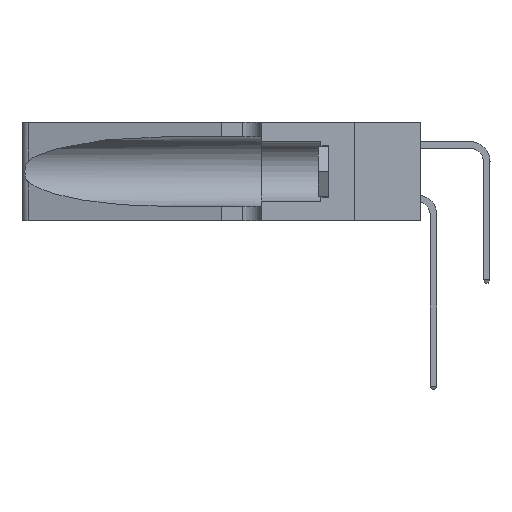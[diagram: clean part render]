
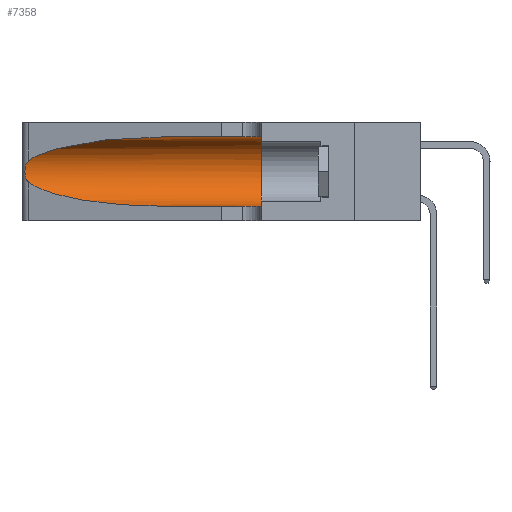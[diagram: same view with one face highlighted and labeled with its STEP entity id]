
A CAD part, left-side view. The second image highlights one B-rep face of the part: STEP entity #7358.
In plain terms, the highlighted cylindrical face has radius 3.308 mm (diameter 6.617 mm), a partial arc.
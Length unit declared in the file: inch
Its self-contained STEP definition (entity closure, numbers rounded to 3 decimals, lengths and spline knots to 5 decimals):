
#191 = ORIENTED_EDGE ( 'NONE', *, *, #30426, .T. ) ;
#884 = ORIENTED_EDGE ( 'NONE', *, *, #35435, .T. ) ;
#1092 = CARTESIAN_POINT ( 'NONE',  ( 0.25856, 1.23593, 0.16098 ) ) ;
#1130 = LINE ( 'NONE', #33942, #11367 ) ;
#1368 = LINE ( 'NONE', #7147, #33151 ) ;
#1555 = DIRECTION ( 'NONE',  ( 0., -1., 0. ) ) ;
#2728 = CYLINDRICAL_SURFACE ( 'NONE', #17965, 0.13025 ) ;
#3986 = CARTESIAN_POINT ( 'NONE',  ( 0.18966, 0.96281, 0.05475 ) ) ;
#5054 = EDGE_LOOP ( 'NONE', ( #191, #884, #16567, #29701, #20101, #30596 ) ) ;
#5937 = CIRCLE ( 'NONE', #17934, 0.13025 ) ;
#7131 = VERTEX_POINT ( 'NONE', #27624 ) ;
#7147 = CARTESIAN_POINT ( 'NONE',  ( 0.1305, 1.61858, 0.05475 ) ) ;
#7358 = ADVANCED_FACE ( 'NONE', ( #21085 ), #2728, .F. ) ;
#7449 = CARTESIAN_POINT ( 'NONE',  ( 0.2373, 1.15595, 0.08982 ) ) ;
#9213 =( BOUNDED_CURVE ( )  B_SPLINE_CURVE ( 3, ( #38783, #7449, #3986, #41925 ),
 .UNSPECIFIED., .F., .F. ) 
 B_SPLINE_CURVE_WITH_KNOTS ( ( 4, 4 ),
 ( 3.44316, 4.71239 ),
 .UNSPECIFIED. ) 
 CURVE ( )  GEOMETRIC_REPRESENTATION_ITEM ( )  RATIONAL_B_SPLINE_CURVE ( ( 1., 0.87, 0.87, 1. ) ) 
 REPRESENTATION_ITEM ( '' )  );
#9512 = DIRECTION ( 'NONE',  ( 0., 1., 0. ) ) ;
#11367 = VECTOR ( 'NONE', #26841, 39.37008 ) ;
#11779 = CARTESIAN_POINT ( 'NONE',  ( 0.25789, 1.23486, 0.15765 ) ) ;
#11877 = B_SPLINE_CURVE_WITH_KNOTS ( 'NONE', 3,
 ( #24388, #38260, #38575, #17968, #38730, #18113, #17671, #42181, #21100, #1092, #11779, #25757, #35576, #42627 ),
 .UNSPECIFIED., .F., .F.,
 ( 4, 2, 2, 2, 2, 2, 4 ),
 ( 0., 0.00027, 0.00053, 0.00107, 0.0016, 0.00187, 0.00214 ),
 .UNSPECIFIED. ) ;
#12684 = EDGE_CURVE ( 'NONE', #18525, #7131, #9213, .T. ) ;
#16567 = ORIENTED_EDGE ( 'NONE', *, *, #12684, .T. ) ;
#16637 = CARTESIAN_POINT ( 'NONE',  ( 0.18966, 0.96281, 0.31525 ) ) ;
#17388 = CARTESIAN_POINT ( 'NONE',  ( 0.25487, 1.22718, 0.22369 ) ) ;
#17671 = CARTESIAN_POINT ( 'NONE',  ( 0.26075, 1.23896, 0.19203 ) ) ;
#17934 = AXIS2_PLACEMENT_3D ( 'NONE', #23655, #9512, #23350 ) ;
#17965 = AXIS2_PLACEMENT_3D ( 'NONE', #39500, #1555, #42969 ) ;
#17968 = CARTESIAN_POINT ( 'NONE',  ( 0.25787, 1.23484, 0.2124 ) ) ;
#18113 = CARTESIAN_POINT ( 'NONE',  ( 0.26018, 1.23835, 0.19895 ) ) ;
#18525 = VERTEX_POINT ( 'NONE', #30726 ) ;
#20101 = ORIENTED_EDGE ( 'NONE', *, *, #28660, .F. ) ;
#21085 = FACE_OUTER_BOUND ( 'NONE', #5054, .T. ) ;
#21093 = EDGE_CURVE ( 'NONE', #7131, #40028, #1368, .T. ) ;
#21100 = CARTESIAN_POINT ( 'NONE',  ( 0.26017, 1.23833, 0.17102 ) ) ;
#23350 = DIRECTION ( 'NONE',  ( 0., 0., 1. ) ) ;
#23655 = CARTESIAN_POINT ( 'NONE',  ( 0.1305, 0.35, 0.185 ) ) ;
#23935 = VERTEX_POINT ( 'NONE', #41813 ) ;
#24388 = CARTESIAN_POINT ( 'NONE',  ( 0.25487, 1.22718, 0.22369 ) ) ;
#25757 = CARTESIAN_POINT ( 'NONE',  ( 0.25639, 1.23186, 0.15144 ) ) ;
#26841 = DIRECTION ( 'NONE',  ( 0., -1., 0. ) ) ;
#27624 = CARTESIAN_POINT ( 'NONE',  ( 0.1305, 0.72297, 0.05475 ) ) ;
#28623 = EDGE_CURVE ( 'NONE', #23935, #43153, #1130, .T. ) ;
#28660 = EDGE_CURVE ( 'NONE', #43153, #40028, #5937, .T. ) ;
#29701 = ORIENTED_EDGE ( 'NONE', *, *, #21093, .T. ) ;
#30426 = EDGE_CURVE ( 'NONE', #23935, #38557, #41114, .T. ) ;
#30596 = ORIENTED_EDGE ( 'NONE', *, *, #28623, .F. ) ;
#30726 = CARTESIAN_POINT ( 'NONE',  ( 0.25487, 1.22718, 0.14631 ) ) ;
#30942 = DIRECTION ( 'NONE',  ( 0., -1., 0. ) ) ;
#33151 = VECTOR ( 'NONE', #30942, 39.37008 ) ;
#33942 = CARTESIAN_POINT ( 'NONE',  ( 0.1305, 1.61858, 0.31525 ) ) ;
#35435 = EDGE_CURVE ( 'NONE', #38557, #18525, #11877, .T. ) ;
#35576 = CARTESIAN_POINT ( 'NONE',  ( 0.25555, 1.22993, 0.14849 ) ) ;
#35728 = CARTESIAN_POINT ( 'NONE',  ( 0.1305, 0.35, 0.05475 ) ) ;
#37230 = CARTESIAN_POINT ( 'NONE',  ( 0.1305, 0.72297, 0.31525 ) ) ;
#37690 = CARTESIAN_POINT ( 'NONE',  ( 0.2373, 1.15595, 0.28018 ) ) ;
#38260 = CARTESIAN_POINT ( 'NONE',  ( 0.25555, 1.22994, 0.2215 ) ) ;
#38557 = VERTEX_POINT ( 'NONE', #39441 ) ;
#38575 = CARTESIAN_POINT ( 'NONE',  ( 0.25639, 1.23184, 0.21858 ) ) ;
#38730 = CARTESIAN_POINT ( 'NONE',  ( 0.25854, 1.2359, 0.20912 ) ) ;
#38783 = CARTESIAN_POINT ( 'NONE',  ( 0.25487, 1.22718, 0.14631 ) ) ;
#39441 = CARTESIAN_POINT ( 'NONE',  ( 0.25487, 1.22718, 0.22369 ) ) ;
#39500 = CARTESIAN_POINT ( 'NONE',  ( 0.1305, 1.61858, 0.185 ) ) ;
#40028 = VERTEX_POINT ( 'NONE', #35728 ) ;
#41114 =( BOUNDED_CURVE ( )  B_SPLINE_CURVE ( 3, ( #37230, #16637, #37690, #17388 ),
 .UNSPECIFIED., .F., .T. ) 
 B_SPLINE_CURVE_WITH_KNOTS ( ( 4, 4 ),
 ( 1.5708, 2.84003 ),
 .UNSPECIFIED. ) 
 CURVE ( )  GEOMETRIC_REPRESENTATION_ITEM ( )  RATIONAL_B_SPLINE_CURVE ( ( 1., 0.87, 0.87, 1. ) ) 
 REPRESENTATION_ITEM ( '' )  );
#41813 = CARTESIAN_POINT ( 'NONE',  ( 0.1305, 0.72297, 0.31525 ) ) ;
#41925 = CARTESIAN_POINT ( 'NONE',  ( 0.1305, 0.72297, 0.05475 ) ) ;
#42181 = CARTESIAN_POINT ( 'NONE',  ( 0.26075, 1.23896, 0.178 ) ) ;
#42627 = CARTESIAN_POINT ( 'NONE',  ( 0.25487, 1.22718, 0.14631 ) ) ;
#42969 = DIRECTION ( 'NONE',  ( 0., 0., -1. ) ) ;
#43153 = VERTEX_POINT ( 'NONE', #43857 ) ;
#43857 = CARTESIAN_POINT ( 'NONE',  ( 0.1305, 0.35, 0.31525 ) ) ;
